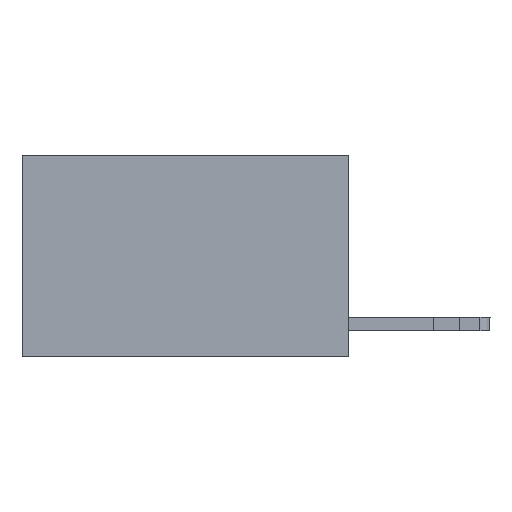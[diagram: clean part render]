
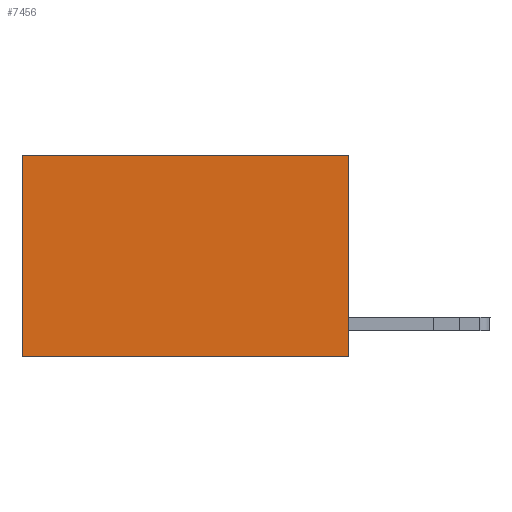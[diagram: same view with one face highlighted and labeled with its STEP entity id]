
A CAD part, left-side view. The second image highlights one B-rep face of the part: STEP entity #7456.
In plain terms, the highlighted planar face has unit normal (-1, 0, 0).
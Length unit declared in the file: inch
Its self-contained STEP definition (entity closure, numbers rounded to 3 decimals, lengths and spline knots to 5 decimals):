
#330 = LINE ( 'NONE', #10894, #9617 ) ;
#404 = DIRECTION ( 'NONE',  ( 0., 0., -1. ) ) ;
#410 = LINE ( 'NONE', #5351, #13305 ) ;
#1471 = EDGE_CURVE ( 'NONE', #15709, #4146, #410, .T. ) ;
#1611 = CARTESIAN_POINT ( 'NONE',  ( 0.2625, 0.6, 0. ) ) ;
#1656 = VERTEX_POINT ( 'NONE', #4786 ) ;
#2105 = DIRECTION ( 'NONE',  ( 0., 1., 0. ) ) ;
#2177 = LINE ( 'NONE', #15227, #14550 ) ;
#2382 = ORIENTED_EDGE ( 'NONE', *, *, #1471, .T. ) ;
#3061 = CARTESIAN_POINT ( 'NONE',  ( 0.2625, 0.6, 0. ) ) ;
#3500 = ORIENTED_EDGE ( 'NONE', *, *, #4370, .F. ) ;
#4146 = VERTEX_POINT ( 'NONE', #1611 ) ;
#4370 = EDGE_CURVE ( 'NONE', #1656, #10902, #330, .T. ) ;
#4786 = CARTESIAN_POINT ( 'NONE',  ( 0.2625, 0., -0.37 ) ) ;
#5351 = CARTESIAN_POINT ( 'NONE',  ( 0.2625, 0., 0. ) ) ;
#5446 = DIRECTION ( 'NONE',  ( 1., 0., 0. ) ) ;
#5745 = EDGE_CURVE ( 'NONE', #15709, #1656, #2177, .T. ) ;
#5998 = ORIENTED_EDGE ( 'NONE', *, *, #14216, .T. ) ;
#6644 = LINE ( 'NONE', #3061, #10038 ) ;
#7456 = ADVANCED_FACE ( 'NONE', ( #11510 ), #10458, .F. ) ;
#8406 = CARTESIAN_POINT ( 'NONE',  ( 0.2625, 0., 0. ) ) ;
#9617 = VECTOR ( 'NONE', #2105, 39.37008 ) ;
#10038 = VECTOR ( 'NONE', #11738, 39.37008 ) ;
#10458 = PLANE ( 'NONE',  #13508 ) ;
#10894 = CARTESIAN_POINT ( 'NONE',  ( 0.2625, 0., -0.37 ) ) ;
#10902 = VERTEX_POINT ( 'NONE', #14068 ) ;
#10934 = DIRECTION ( 'NONE',  ( 0., 1., 0. ) ) ;
#11510 = FACE_OUTER_BOUND ( 'NONE', #14675, .T. ) ;
#11738 = DIRECTION ( 'NONE',  ( 0., 0., -1. ) ) ;
#12889 = CARTESIAN_POINT ( 'NONE',  ( 0.2625, 0., 0. ) ) ;
#13305 = VECTOR ( 'NONE', #10934, 39.37008 ) ;
#13508 = AXIS2_PLACEMENT_3D ( 'NONE', #12889, #5446, #14060 ) ;
#14060 = DIRECTION ( 'NONE',  ( 0., 0., -1. ) ) ;
#14068 = CARTESIAN_POINT ( 'NONE',  ( 0.2625, 0.6, -0.37 ) ) ;
#14216 = EDGE_CURVE ( 'NONE', #4146, #10902, #6644, .T. ) ;
#14550 = VECTOR ( 'NONE', #404, 39.37008 ) ;
#14675 = EDGE_LOOP ( 'NONE', ( #5998, #3500, #15075, #2382 ) ) ;
#15075 = ORIENTED_EDGE ( 'NONE', *, *, #5745, .F. ) ;
#15227 = CARTESIAN_POINT ( 'NONE',  ( 0.2625, 0., 0. ) ) ;
#15709 = VERTEX_POINT ( 'NONE', #8406 ) ;
